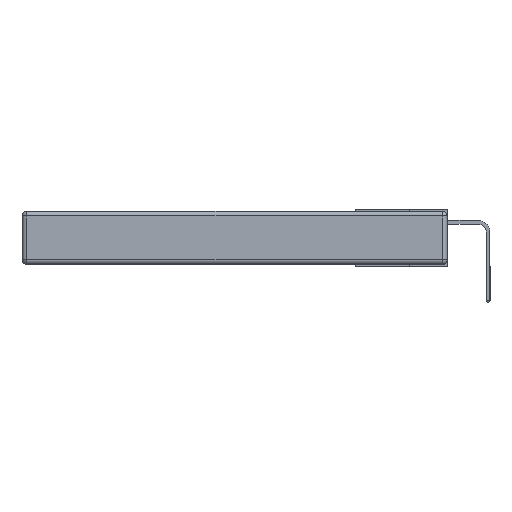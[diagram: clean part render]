
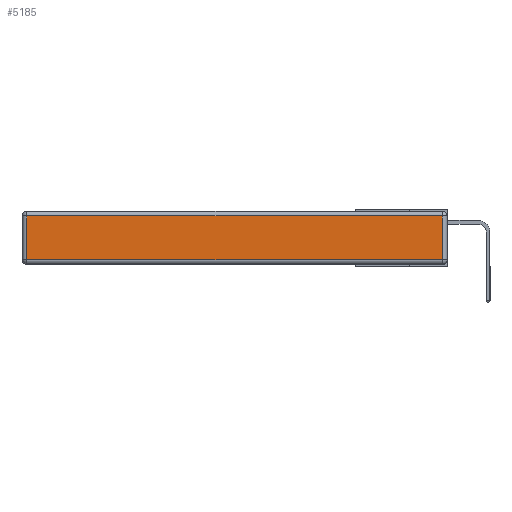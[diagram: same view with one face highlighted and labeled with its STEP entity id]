
A CAD part, left-side view. The second image highlights one B-rep face of the part: STEP entity #5185.
In plain terms, the highlighted planar face has unit normal (-1, 0, 0).
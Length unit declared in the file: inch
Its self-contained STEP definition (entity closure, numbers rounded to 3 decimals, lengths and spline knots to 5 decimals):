
#817 = EDGE_CURVE ( 'NONE', #14809, #9024, #7085, .T. ) ;
#1080 = CARTESIAN_POINT ( 'NONE',  ( 0., 0., -0.313 ) ) ;
#1252 = DIRECTION ( 'NONE',  ( 0., 0., 1. ) ) ;
#1904 = VECTOR ( 'NONE', #15460, 39.37008 ) ;
#2858 = CARTESIAN_POINT ( 'NONE',  ( 0., 2.72, -0.313 ) ) ;
#4298 = DIRECTION ( 'NONE',  ( 0., 0., 1. ) ) ;
#4373 = VERTEX_POINT ( 'NONE', #2858 ) ;
#4743 = DIRECTION ( 'NONE',  ( 0., 1., 0. ) ) ;
#4895 = EDGE_LOOP ( 'NONE', ( #7786, #12045, #12709, #5909 ) ) ;
#5085 = CARTESIAN_POINT ( 'NONE',  ( 0., 0.03, -0.313 ) ) ;
#5185 = ADVANCED_FACE ( 'NONE', ( #9800 ), #11442, .T. ) ;
#5481 = VECTOR ( 'NONE', #1252, 39.37008 ) ;
#5787 = CARTESIAN_POINT ( 'NONE',  ( 0., 0.03, -0.03 ) ) ;
#5885 = VERTEX_POINT ( 'NONE', #5085 ) ;
#5909 = ORIENTED_EDGE ( 'NONE', *, *, #8512, .T. ) ;
#6313 = EDGE_CURVE ( 'NONE', #4373, #5885, #9870, .T. ) ;
#6622 = DIRECTION ( 'NONE',  ( -1., 0., 0. ) ) ;
#6784 = CARTESIAN_POINT ( 'NONE',  ( 0., 0., -0.343 ) ) ;
#7085 = LINE ( 'NONE', #10817, #8999 ) ;
#7444 = CARTESIAN_POINT ( 'NONE',  ( 0., 2.72, -0.343 ) ) ;
#7786 = ORIENTED_EDGE ( 'NONE', *, *, #6313, .T. ) ;
#8512 = EDGE_CURVE ( 'NONE', #9024, #4373, #10184, .T. ) ;
#8999 = VECTOR ( 'NONE', #4743, 39.37008 ) ;
#9024 = VERTEX_POINT ( 'NONE', #14339 ) ;
#9099 = LINE ( 'NONE', #9662, #5481 ) ;
#9662 = CARTESIAN_POINT ( 'NONE',  ( 0., 0.03, -0.343 ) ) ;
#9800 = FACE_OUTER_BOUND ( 'NONE', #4895, .T. ) ;
#9870 = LINE ( 'NONE', #1080, #1904 ) ;
#10184 = LINE ( 'NONE', #7444, #14515 ) ;
#10769 = AXIS2_PLACEMENT_3D ( 'NONE', #6784, #6622, #4298 ) ;
#10817 = CARTESIAN_POINT ( 'NONE',  ( 0., 2.75, -0.03 ) ) ;
#11442 = PLANE ( 'NONE',  #10769 ) ;
#12045 = ORIENTED_EDGE ( 'NONE', *, *, #14104, .T. ) ;
#12709 = ORIENTED_EDGE ( 'NONE', *, *, #817, .T. ) ;
#13519 = DIRECTION ( 'NONE',  ( 0., 0., -1. ) ) ;
#14104 = EDGE_CURVE ( 'NONE', #5885, #14809, #9099, .T. ) ;
#14339 = CARTESIAN_POINT ( 'NONE',  ( 0., 2.72, -0.03 ) ) ;
#14515 = VECTOR ( 'NONE', #13519, 39.37008 ) ;
#14809 = VERTEX_POINT ( 'NONE', #5787 ) ;
#15460 = DIRECTION ( 'NONE',  ( 0., -1., 0. ) ) ;
